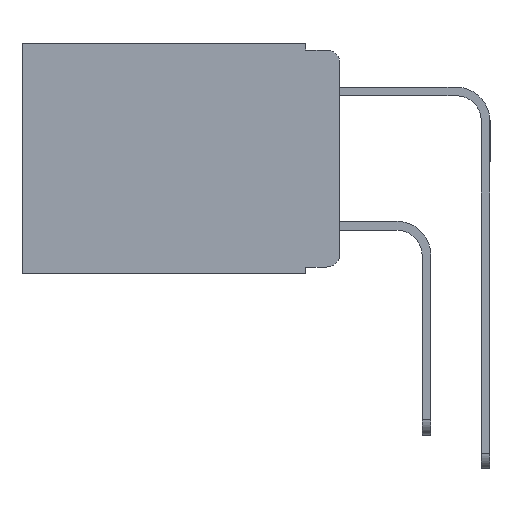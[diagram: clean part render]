
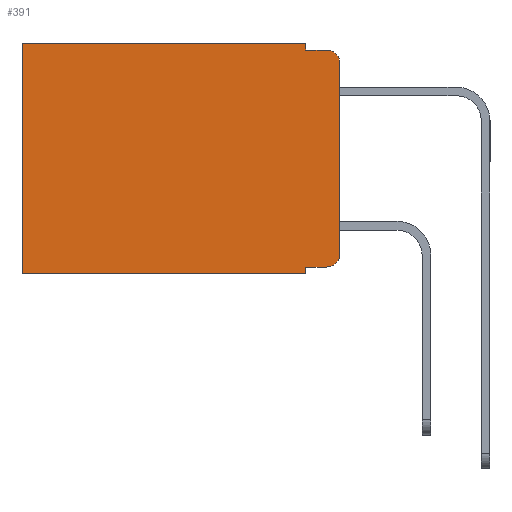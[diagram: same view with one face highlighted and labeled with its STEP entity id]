
A CAD part, left-side view. The second image highlights one B-rep face of the part: STEP entity #391.
In plain terms, the highlighted planar face has unit normal (-1, 0, 0).
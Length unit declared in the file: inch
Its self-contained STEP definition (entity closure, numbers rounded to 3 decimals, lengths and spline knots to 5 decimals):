
#242 = ORIENTED_EDGE ( 'NONE', *, *, #10602, .F. ) ;
#387 = DIRECTION ( 'NONE',  ( -1., 0., 0. ) ) ;
#391 = ADVANCED_FACE ( 'NONE', ( #2234 ), #9490, .F. ) ;
#400 = DIRECTION ( 'NONE',  ( 0., 0., -1. ) ) ;
#418 = EDGE_CURVE ( 'NONE', #10302, #7488, #4028, .T. ) ;
#554 = CARTESIAN_POINT ( 'NONE',  ( 0.298, 0.051, -0.333 ) ) ;
#755 = DIRECTION ( 'NONE',  ( 0., 0., -1. ) ) ;
#790 = ORIENTED_EDGE ( 'NONE', *, *, #2666, .T. ) ;
#903 = CARTESIAN_POINT ( 'NONE',  ( 0.298, 0.051, -0.333 ) ) ;
#1121 = CARTESIAN_POINT ( 'NONE',  ( 0.298, 0., 0. ) ) ;
#1160 = CARTESIAN_POINT ( 'NONE',  ( 0.298, 0., -0.03 ) ) ;
#1270 = CARTESIAN_POINT ( 'NONE',  ( 0.298, 0.02, -0.03 ) ) ;
#1290 = CARTESIAN_POINT ( 'NONE',  ( 0.298, 0., 0. ) ) ;
#1317 = VERTEX_POINT ( 'NONE', #554 ) ;
#1440 = EDGE_CURVE ( 'NONE', #5641, #1707, #9463, .T. ) ;
#1494 = LINE ( 'NONE', #3351, #7917 ) ;
#1707 = VERTEX_POINT ( 'NONE', #9155 ) ;
#1808 = AXIS2_PLACEMENT_3D ( 'NONE', #1270, #8524, #8582 ) ;
#1945 = DIRECTION ( 'NONE',  ( 0., -1., 0. ) ) ;
#1997 = ORIENTED_EDGE ( 'NONE', *, *, #2486, .T. ) ;
#2011 = ORIENTED_EDGE ( 'NONE', *, *, #10954, .T. ) ;
#2104 = CARTESIAN_POINT ( 'NONE',  ( 0.298, 0.473, -0.343 ) ) ;
#2234 = FACE_OUTER_BOUND ( 'NONE', #9953, .T. ) ;
#2258 = CARTESIAN_POINT ( 'NONE',  ( 0.298, 0.02, -0.333 ) ) ;
#2259 = CARTESIAN_POINT ( 'NONE',  ( 0.298, 0.051, -0.343 ) ) ;
#2486 = EDGE_CURVE ( 'NONE', #3462, #7488, #6317, .T. ) ;
#2631 = VECTOR ( 'NONE', #11264, 39.37008 ) ;
#2666 = EDGE_CURVE ( 'NONE', #1707, #4196, #6043, .T. ) ;
#3166 = DIRECTION ( 'NONE',  ( 0., 0., -1. ) ) ;
#3234 = CARTESIAN_POINT ( 'NONE',  ( 0.298, 0., 0. ) ) ;
#3351 = CARTESIAN_POINT ( 'NONE',  ( 0.298, 0.051, -0.01 ) ) ;
#3435 = VERTEX_POINT ( 'NONE', #4895 ) ;
#3462 = VERTEX_POINT ( 'NONE', #2258 ) ;
#3529 = ORIENTED_EDGE ( 'NONE', *, *, #1440, .T. ) ;
#3561 = ORIENTED_EDGE ( 'NONE', *, *, #4677, .F. ) ;
#3799 = CARTESIAN_POINT ( 'NONE',  ( 0.298, 0., -0.343 ) ) ;
#3952 = CARTESIAN_POINT ( 'NONE',  ( 0.298, 0.051, -0.01 ) ) ;
#4028 = LINE ( 'NONE', #1121, #2631 ) ;
#4196 = VERTEX_POINT ( 'NONE', #2104 ) ;
#4244 = EDGE_CURVE ( 'NONE', #10740, #4196, #7518, .T. ) ;
#4480 = LINE ( 'NONE', #903, #6784 ) ;
#4669 = VECTOR ( 'NONE', #3166, 39.37008 ) ;
#4677 = EDGE_CURVE ( 'NONE', #1317, #10740, #8504, .T. ) ;
#4895 = CARTESIAN_POINT ( 'NONE',  ( 0.298, 0.02, -0.01 ) ) ;
#5426 = CIRCLE ( 'NONE', #1808, 0.02 ) ;
#5641 = VERTEX_POINT ( 'NONE', #11434 ) ;
#5711 = ORIENTED_EDGE ( 'NONE', *, *, #418, .F. ) ;
#5719 = VECTOR ( 'NONE', #10782, 39.37008 ) ;
#5960 = DIRECTION ( 'NONE',  ( 0., 1., 0. ) ) ;
#6043 = LINE ( 'NONE', #8048, #7770 ) ;
#6317 = CIRCLE ( 'NONE', #8777, 0.02 ) ;
#6470 = VECTOR ( 'NONE', #5960, 39.37008 ) ;
#6784 = VECTOR ( 'NONE', #1945, 39.37008 ) ;
#6812 = DIRECTION ( 'NONE',  ( 0., 0., -1. ) ) ;
#7488 = VERTEX_POINT ( 'NONE', #7599 ) ;
#7518 = LINE ( 'NONE', #3799, #9968 ) ;
#7592 = DIRECTION ( 'NONE',  ( 1., 0., 0. ) ) ;
#7599 = CARTESIAN_POINT ( 'NONE',  ( 0.298, 0., -0.313 ) ) ;
#7762 = AXIS2_PLACEMENT_3D ( 'NONE', #1290, #7592, #400 ) ;
#7770 = VECTOR ( 'NONE', #755, 39.37008 ) ;
#7917 = VECTOR ( 'NONE', #8742, 39.37008 ) ;
#8048 = CARTESIAN_POINT ( 'NONE',  ( 0.298, 0.473, 0. ) ) ;
#8107 = LINE ( 'NONE', #11727, #5719 ) ;
#8504 = LINE ( 'NONE', #11352, #4669 ) ;
#8524 = DIRECTION ( 'NONE',  ( -1., 0., 0. ) ) ;
#8582 = DIRECTION ( 'NONE',  ( 0., 0., -1. ) ) ;
#8642 = ORIENTED_EDGE ( 'NONE', *, *, #9700, .T. ) ;
#8742 = DIRECTION ( 'NONE',  ( 0., -1., 0. ) ) ;
#8777 = AXIS2_PLACEMENT_3D ( 'NONE', #9479, #387, #6812 ) ;
#9155 = CARTESIAN_POINT ( 'NONE',  ( 0.298, 0.473, 0. ) ) ;
#9463 = LINE ( 'NONE', #3234, #6470 ) ;
#9479 = CARTESIAN_POINT ( 'NONE',  ( 0.298, 0.02, -0.313 ) ) ;
#9490 = PLANE ( 'NONE',  #7762 ) ;
#9700 = EDGE_CURVE ( 'NONE', #10302, #3435, #5426, .T. ) ;
#9953 = EDGE_LOOP ( 'NONE', ( #5711, #8642, #11700, #242, #3529, #790, #11021, #3561, #2011, #1997 ) ) ;
#9968 = VECTOR ( 'NONE', #11025, 39.37008 ) ;
#10247 = VERTEX_POINT ( 'NONE', #3952 ) ;
#10302 = VERTEX_POINT ( 'NONE', #1160 ) ;
#10602 = EDGE_CURVE ( 'NONE', #5641, #10247, #8107, .T. ) ;
#10740 = VERTEX_POINT ( 'NONE', #2259 ) ;
#10782 = DIRECTION ( 'NONE',  ( 0., 0., -1. ) ) ;
#10918 = EDGE_CURVE ( 'NONE', #10247, #3435, #1494, .T. ) ;
#10954 = EDGE_CURVE ( 'NONE', #1317, #3462, #4480, .T. ) ;
#11021 = ORIENTED_EDGE ( 'NONE', *, *, #4244, .F. ) ;
#11025 = DIRECTION ( 'NONE',  ( 0., 1., 0. ) ) ;
#11264 = DIRECTION ( 'NONE',  ( 0., 0., -1. ) ) ;
#11352 = CARTESIAN_POINT ( 'NONE',  ( 0.298, 0.051, 0. ) ) ;
#11434 = CARTESIAN_POINT ( 'NONE',  ( 0.298, 0.051, 0. ) ) ;
#11700 = ORIENTED_EDGE ( 'NONE', *, *, #10918, .F. ) ;
#11727 = CARTESIAN_POINT ( 'NONE',  ( 0.298, 0.051, 0. ) ) ;
